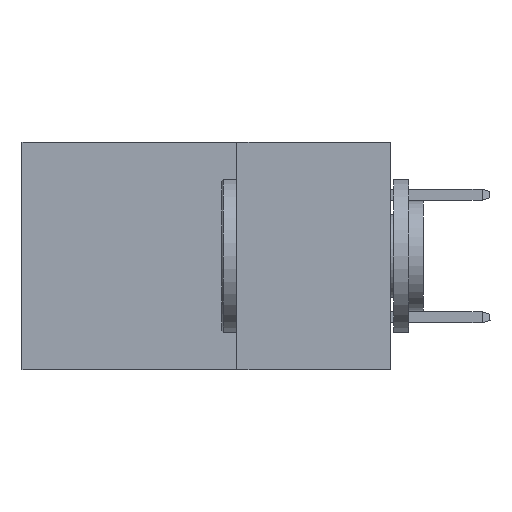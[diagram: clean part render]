
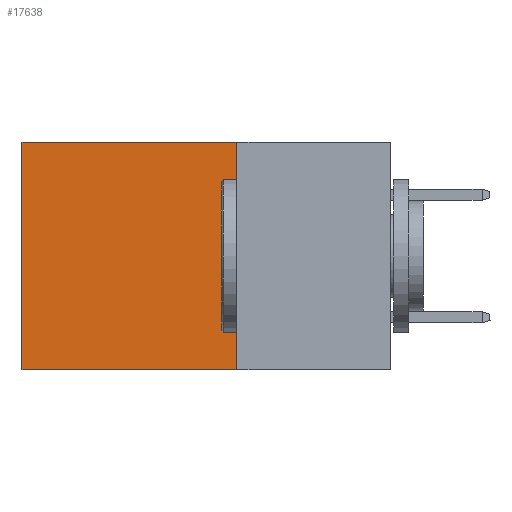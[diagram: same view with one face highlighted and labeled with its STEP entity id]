
A CAD part, left-side view. The second image highlights one B-rep face of the part: STEP entity #17638.
In plain terms, the highlighted planar face has unit normal (-1, 0, 0).
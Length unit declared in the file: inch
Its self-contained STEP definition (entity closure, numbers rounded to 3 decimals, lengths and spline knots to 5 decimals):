
#328 = EDGE_CURVE ( 'NONE', #15143, #16492, #16910, .T. ) ;
#1391 = FACE_OUTER_BOUND ( 'NONE', #2611, .T. ) ;
#1670 = CARTESIAN_POINT ( 'NONE',  ( 0.2875, 0.25, -0.37 ) ) ;
#2564 = VECTOR ( 'NONE', #11732, 39.37008 ) ;
#2611 = EDGE_LOOP ( 'NONE', ( #21064, #4849, #17588, #10811 ) ) ;
#2697 = VECTOR ( 'NONE', #15834, 39.37008 ) ;
#3320 = CARTESIAN_POINT ( 'NONE',  ( 0.2875, 0.25, 0. ) ) ;
#3358 = CARTESIAN_POINT ( 'NONE',  ( 0.2875, 0.25, -0.37 ) ) ;
#3415 = DIRECTION ( 'NONE',  ( 0., 1., 0. ) ) ;
#4849 = ORIENTED_EDGE ( 'NONE', *, *, #20030, .F. ) ;
#5079 = DIRECTION ( 'NONE',  ( 0., 0., -1. ) ) ;
#5579 = EDGE_CURVE ( 'NONE', #8714, #15143, #16491, .T. ) ;
#6099 = AXIS2_PLACEMENT_3D ( 'NONE', #3320, #15518, #5079 ) ;
#6277 = VERTEX_POINT ( 'NONE', #3358 ) ;
#8583 = LINE ( 'NONE', #1670, #17354 ) ;
#8714 = VERTEX_POINT ( 'NONE', #15534 ) ;
#8822 = EDGE_CURVE ( 'NONE', #8714, #6277, #16628, .T. ) ;
#8875 = CARTESIAN_POINT ( 'NONE',  ( 0.2875, 0.6, 0. ) ) ;
#10811 = ORIENTED_EDGE ( 'NONE', *, *, #5579, .T. ) ;
#11686 = VECTOR ( 'NONE', #19752, 39.37008 ) ;
#11732 = DIRECTION ( 'NONE',  ( 0., 1., 0. ) ) ;
#12511 = CARTESIAN_POINT ( 'NONE',  ( 0.2875, 0.6, -0.37 ) ) ;
#14076 = CARTESIAN_POINT ( 'NONE',  ( 0.2875, 0.25, 0. ) ) ;
#15143 = VERTEX_POINT ( 'NONE', #8875 ) ;
#15207 = CARTESIAN_POINT ( 'NONE',  ( 0.2875, 0.25, 0. ) ) ;
#15518 = DIRECTION ( 'NONE',  ( 1., 0., 0. ) ) ;
#15534 = CARTESIAN_POINT ( 'NONE',  ( 0.2875, 0.25, 0. ) ) ;
#15834 = DIRECTION ( 'NONE',  ( 0., 0., -1. ) ) ;
#16491 = LINE ( 'NONE', #15207, #2564 ) ;
#16492 = VERTEX_POINT ( 'NONE', #12511 ) ;
#16628 = LINE ( 'NONE', #14076, #2697 ) ;
#16910 = LINE ( 'NONE', #18406, #11686 ) ;
#17354 = VECTOR ( 'NONE', #3415, 39.37008 ) ;
#17588 = ORIENTED_EDGE ( 'NONE', *, *, #8822, .F. ) ;
#17638 = ADVANCED_FACE ( 'NONE', ( #1391 ), #22391, .F. ) ;
#18406 = CARTESIAN_POINT ( 'NONE',  ( 0.2875, 0.6, 0. ) ) ;
#19752 = DIRECTION ( 'NONE',  ( 0., 0., -1. ) ) ;
#20030 = EDGE_CURVE ( 'NONE', #6277, #16492, #8583, .T. ) ;
#21064 = ORIENTED_EDGE ( 'NONE', *, *, #328, .T. ) ;
#22391 = PLANE ( 'NONE',  #6099 ) ;
